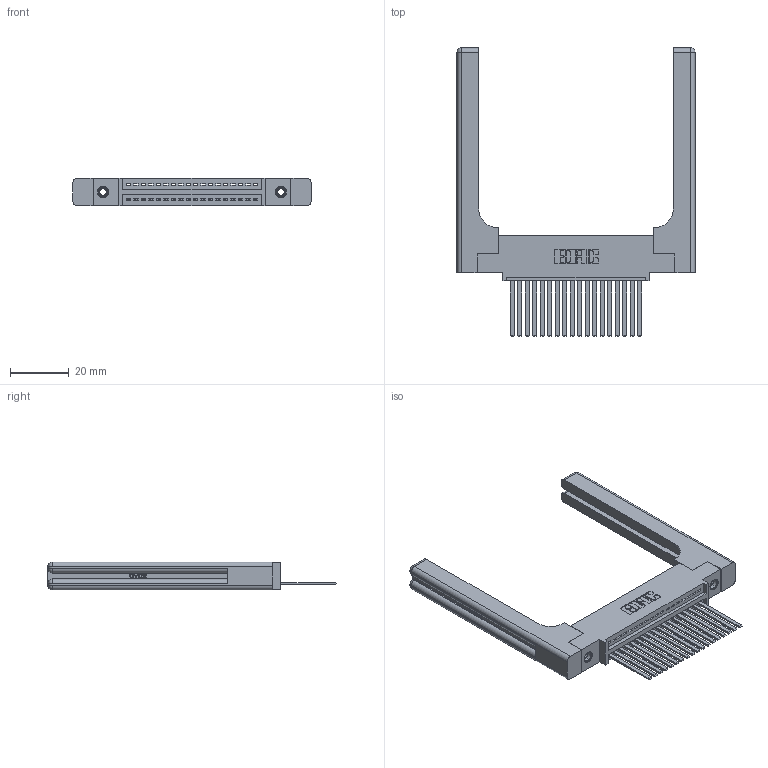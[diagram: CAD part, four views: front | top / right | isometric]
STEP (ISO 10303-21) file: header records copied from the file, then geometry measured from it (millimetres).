
FILE_DESCRIPTION (( 'STEP AP203' ), '1' );
FILE_NAME ('395-018-544-458.STEP', '2019-10-17T16:18:30', ( '' ), ( '' ), 'SwSTEP 2.0', 'SolidWorks 2016', '' );
FILE_SCHEMA (( 'CONFIG_CONTROL_DESIGN' ));
Length unit declared in the file: inch
Products named in the file (5): 345-292-001_345-293-144; 345 Part_0.110 Offset - 0.156 Dia-TH; 395-018-544-458; 345-220-058_345-220-058; 345-250-001_345-250-001-102
Assembly tree (23 placements, depth 2):
  395-018-544-458
    345 Part_0.110 Offset - 0.156 Dia-TH
    345-292-001_345-293-144  x18
    345-250-001_345-250-001-102  x2
    345-220-058_345-220-058  x2
Bounding box: 80.75 x 97.71 x 9.4 mm (x, y, z)
Volume: 16112.9 mm3; surface area: 15797.3 mm2
Topology: 23 solids, 23 shells, 1322 faces, 3863 edges, 2530 vertices
Faces by surface type: plane 880, cylinder 382, bspline 36, cone 12, sphere 8, torus 4
Entity records: 21908 total; most frequent: CARTESIAN_POINT 4767, ORIENTED_EDGE 3516, DIRECTION 3142, EDGE_CURVE 1758, LINE 1466, VECTOR 1466, VERTEX_POINT 1162, AXIS2_PLACEMENT_3D 838
